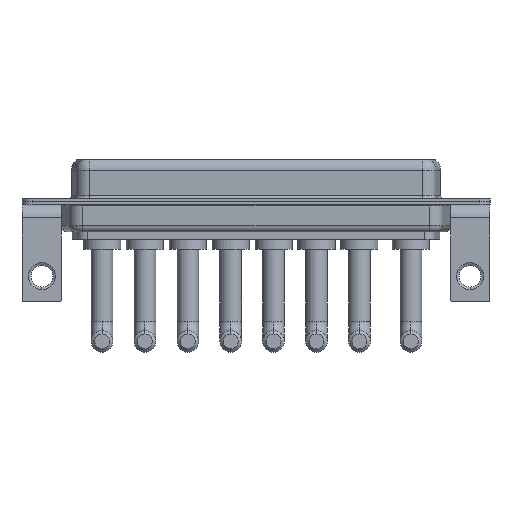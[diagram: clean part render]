
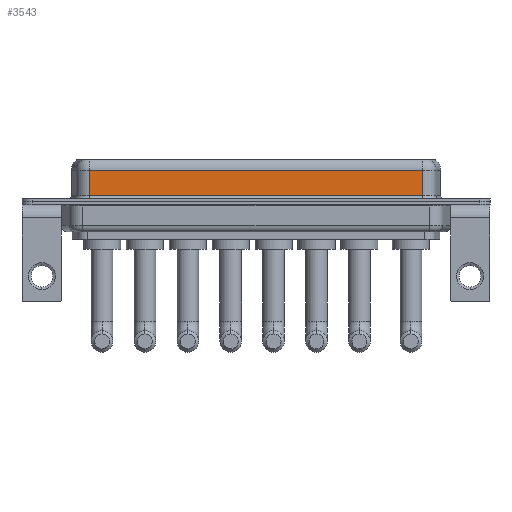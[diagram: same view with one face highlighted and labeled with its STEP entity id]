
A CAD part, front view. The second image highlights one B-rep face of the part: STEP entity #3543.
In plain terms, the highlighted planar face has unit normal (0, -1, 0).
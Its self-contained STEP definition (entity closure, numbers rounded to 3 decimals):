
#381 = CARTESIAN_POINT ( 'NONE',  ( 7.038, -3.95, 0.9 ) ) ;
#528 = CARTESIAN_POINT ( 'NONE',  ( 56.462, -3.95, 4.65 ) ) ;
#979 = VECTOR ( 'NONE', #5404, 1000. ) ;
#1006 = CARTESIAN_POINT ( 'NONE',  ( 56.462, -3.95, 6.4 ) ) ;
#1055 = EDGE_CURVE ( 'NONE', #7130, #4381, #1112, .T. ) ;
#1112 = LINE ( 'NONE', #6399, #979 ) ;
#2495 = EDGE_CURVE ( 'NONE', #13613, #7130, #13641, .T. ) ;
#2893 = ORIENTED_EDGE ( 'NONE', *, *, #12324, .T. ) ;
#3022 = CARTESIAN_POINT ( 'NONE',  ( 56.462, -3.95, 0.9 ) ) ;
#3041 = DIRECTION ( 'NONE',  ( 0., 0., 1. ) ) ;
#3543 = ADVANCED_FACE ( 'NONE', ( #12865 ), #5405, .F. ) ;
#4008 = VERTEX_POINT ( 'NONE', #3022 ) ;
#4072 = VECTOR ( 'NONE', #6918, 1000. ) ;
#4381 = VERTEX_POINT ( 'NONE', #381 ) ;
#5158 = EDGE_LOOP ( 'NONE', ( #13363, #12612, #13320, #2893 ) ) ;
#5230 = DIRECTION ( 'NONE',  ( 0., 0., -1. ) ) ;
#5260 = CARTESIAN_POINT ( 'NONE',  ( 56.462, -3.95, 6.4 ) ) ;
#5404 = DIRECTION ( 'NONE',  ( 0., 0., -1. ) ) ;
#5405 = PLANE ( 'NONE',  #12139 ) ;
#5473 = DIRECTION ( 'NONE',  ( 0., 1., 0. ) ) ;
#6399 = CARTESIAN_POINT ( 'NONE',  ( 7.038, -3.95, 6.4 ) ) ;
#6411 = VECTOR ( 'NONE', #7956, 1000. ) ;
#6876 = CARTESIAN_POINT ( 'NONE',  ( 7.038, -3.95, 4.65 ) ) ;
#6918 = DIRECTION ( 'NONE',  ( 1., 0., 0. ) ) ;
#7084 = CARTESIAN_POINT ( 'NONE',  ( 56.462, -3.95, 4.65 ) ) ;
#7130 = VERTEX_POINT ( 'NONE', #6876 ) ;
#7956 = DIRECTION ( 'NONE',  ( -1., 0., 0. ) ) ;
#9784 = LINE ( 'NONE', #1006, #13404 ) ;
#11126 = LINE ( 'NONE', #13256, #4072 ) ;
#12139 = AXIS2_PLACEMENT_3D ( 'NONE', #5260, #5473, #3041 ) ;
#12270 = EDGE_CURVE ( 'NONE', #13613, #4008, #9784, .T. ) ;
#12324 = EDGE_CURVE ( 'NONE', #4381, #4008, #11126, .T. ) ;
#12612 = ORIENTED_EDGE ( 'NONE', *, *, #2495, .T. ) ;
#12865 = FACE_OUTER_BOUND ( 'NONE', #5158, .T. ) ;
#13256 = CARTESIAN_POINT ( 'NONE',  ( 56.462, -3.95, 0.9 ) ) ;
#13320 = ORIENTED_EDGE ( 'NONE', *, *, #1055, .T. ) ;
#13363 = ORIENTED_EDGE ( 'NONE', *, *, #12270, .F. ) ;
#13404 = VECTOR ( 'NONE', #5230, 1000. ) ;
#13613 = VERTEX_POINT ( 'NONE', #7084 ) ;
#13641 = LINE ( 'NONE', #528, #6411 ) ;
